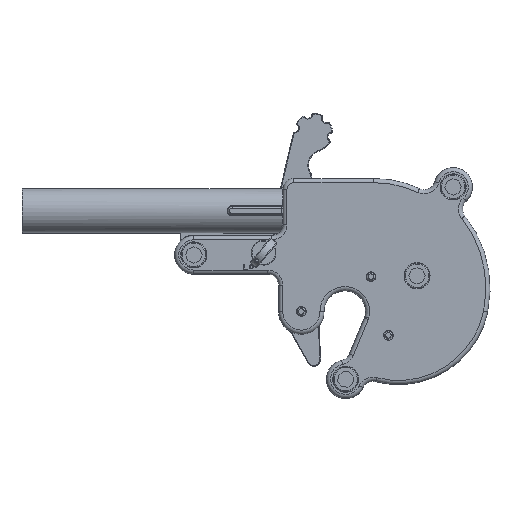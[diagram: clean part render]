
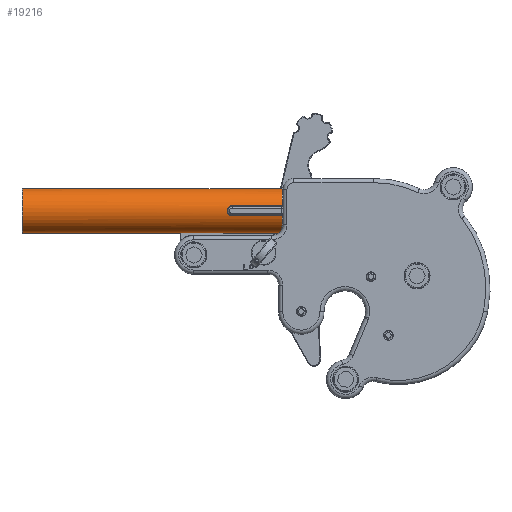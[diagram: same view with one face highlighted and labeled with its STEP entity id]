
A CAD part, top view. The second image highlights one B-rep face of the part: STEP entity #19216.
In plain terms, the highlighted cylindrical face has radius 8.1 mm (diameter 16.2 mm), a partial arc.
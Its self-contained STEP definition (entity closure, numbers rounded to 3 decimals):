
#982=CYLINDRICAL_SURFACE($,#20896,8.1);
#1768=B_SPLINE_CURVE_WITH_KNOTS($,3,(#31391,#31392,#31393,#31394,#31395,
#31396,#31397,#31398),.UNSPECIFIED.,.F.,.F.,(4,1,1,1,1,4),(5.289,
5.588,5.737,6.036,6.111,6.296),
 .UNSPECIFIED.);
#1769=B_SPLINE_CURVE_WITH_KNOTS($,3,(#31400,#31401,#31402,#31403),
 .UNSPECIFIED.,.F.,.F.,(4,4),(6.296,6.3),
 .UNSPECIFIED.);
#1772=B_SPLINE_CURVE_WITH_KNOTS($,3,(#31496,#31497,#31498,#31499,#31500,
#31501,#31502,#31503,#31504,#31505),.UNSPECIFIED.,.F.,.F.,(4,1,1,1,1,1,
1,4),(0.,0.079,0.118,0.236,0.315,
0.394,0.473,0.552),.UNSPECIFIED.);
#1778=B_SPLINE_CURVE_WITH_KNOTS($,3,(#31861,#31862,#31863,#31864,#31865,
#31866),.UNSPECIFIED.,.F.,.F.,(4,2,4),(-0.162,-0.152,
-0.143),.UNSPECIFIED.);
#1779=B_SPLINE_CURVE_WITH_KNOTS($,3,(#31923,#31924,#31925,#31926,#31927,
#31928,#31929,#31930,#31931,#31932),.UNSPECIFIED.,.F.,.F.,(4,2,2,2,4),(0.,
0.,0.04,0.052,0.06),
 .UNSPECIFIED.);
#2176=FACE_OUTER_BOUND($,#3521,.T.);
#3521=EDGE_LOOP($,(#14006,#14007,#14008,#14009,#14010,#14011,#14012,#14013,
#14014,#14015,#14016,#14017,#14018,#14019));
#4990=CIRCLE($,#20615,8.1);
#5063=CIRCLE($,#20723,8.1);
#5080=CIRCLE($,#20748,8.1);
#5157=CIRCLE($,#20886,8.1);
#6527=LINE($,#30896,#7532);
#6555=LINE($,#31431,#7560);
#6557=LINE($,#31507,#7562);
#6607=LINE($,#32069,#7612);
#6608=LINE($,#32071,#7613);
#7532=VECTOR($,#23895,94.5);
#7560=VECTOR($,#24139,18.25);
#7562=VECTOR($,#24145,18.25);
#7612=VECTOR($,#24515,57.073);
#7613=VECTOR($,#24518,36.084);
#8621=VERTEX_POINT($,#30821);
#8622=VERTEX_POINT($,#30825);
#8636=VERTEX_POINT($,#30895);
#8709=VERTEX_POINT($,#31329);
#8712=VERTEX_POINT($,#31336);
#8715=VERTEX_POINT($,#31390);
#8716=VERTEX_POINT($,#31399);
#8719=VERTEX_POINT($,#31421);
#8723=VERTEX_POINT($,#31429);
#8725=VERTEX_POINT($,#31494);
#8766=VERTEX_POINT($,#31855);
#8773=VERTEX_POINT($,#31921);
#8774=VERTEX_POINT($,#31922);
#8791=VERTEX_POINT($,#32056);
#10437=EDGE_CURVE($,#8622,#8621,#4990,.T.);
#10454=EDGE_CURVE($,#8621,#8636,#6527,.T.);
#10565=EDGE_CURVE($,#8709,#8712,#5063,.T.);
#10567=EDGE_CURVE($,#8712,#8715,#1768,.T.);
#10568=EDGE_CURVE($,#8715,#8716,#1769,.T.);
#10577=EDGE_CURVE($,#8723,#8709,#6555,.T.);
#10581=EDGE_CURVE($,#8725,#8723,#1772,.T.);
#10582=EDGE_CURVE($,#8719,#8725,#6557,.T.);
#10592=EDGE_CURVE($,#8636,#8719,#5080,.T.);
#10669=EDGE_CURVE($,#8716,#8766,#1778,.T.);
#10680=EDGE_CURVE($,#8773,#8774,#1779,.F.);
#10729=EDGE_CURVE($,#8774,#8791,#5157,.T.);
#10736=EDGE_CURVE($,#8622,#8791,#6607,.T.);
#10737=EDGE_CURVE($,#8773,#8766,#6608,.T.);
#14006=ORIENTED_EDGE($,*,*,#10437,.F.);
#14007=ORIENTED_EDGE($,*,*,#10736,.T.);
#14008=ORIENTED_EDGE($,*,*,#10729,.F.);
#14009=ORIENTED_EDGE($,*,*,#10680,.F.);
#14010=ORIENTED_EDGE($,*,*,#10737,.T.);
#14011=ORIENTED_EDGE($,*,*,#10669,.F.);
#14012=ORIENTED_EDGE($,*,*,#10568,.F.);
#14013=ORIENTED_EDGE($,*,*,#10567,.F.);
#14014=ORIENTED_EDGE($,*,*,#10565,.F.);
#14015=ORIENTED_EDGE($,*,*,#10577,.F.);
#14016=ORIENTED_EDGE($,*,*,#10581,.F.);
#14017=ORIENTED_EDGE($,*,*,#10582,.F.);
#14018=ORIENTED_EDGE($,*,*,#10592,.F.);
#14019=ORIENTED_EDGE($,*,*,#10454,.F.);
#19216=ADVANCED_FACE($,(#2176),#982,.T.);
#20615=AXIS2_PLACEMENT_3D($,#30827,#23868,#23869);
#20723=AXIS2_PLACEMENT_3D($,#31340,#24117,#24118);
#20748=AXIS2_PLACEMENT_3D($,#31525,#24171,#24172);
#20886=AXIS2_PLACEMENT_3D($,#32057,#24495,#24496);
#20896=AXIS2_PLACEMENT_3D($,#32070,#24516,#24517);
#23868=DIRECTION('center_axis',(0.,0.,-1.));
#23869=DIRECTION('ref_axis',(-0.998,-0.067,0.));
#23895=DIRECTION($,(0.,0.,1.));
#24117=DIRECTION('center_axis',(0.,0.,1.));
#24118=DIRECTION('ref_axis',(-0.908,-0.419,0.));
#24139=DIRECTION($,(0.,0.,1.));
#24145=DIRECTION($,(0.,0.,-1.));
#24171=DIRECTION('center_axis',(0.,0.,1.));
#24172=DIRECTION('ref_axis',(-0.302,0.953,0.));
#24495=DIRECTION('center_axis',(0.,0.,1.));
#24496=DIRECTION('ref_axis',(0.604,-0.797,0.));
#24515=DIRECTION($,(0.,0.,1.));
#24516=DIRECTION('center_axis',(0.,0.,1.));
#24517=DIRECTION('ref_axis',(0.696,0.718,0.));
#24518=DIRECTION($,(0.,0.,1.));
#30821=CARTESIAN_POINT('',(-0.654,7.295,5.25));
#30825=CARTESIAN_POINT('',(0.077,-3.521,5.25));
#30827=CARTESIAN_POINT('Origin',(-6.294,1.481,5.25));
#30895=CARTESIAN_POINT('',(-0.654,7.295,99.75));
#30896=CARTESIAN_POINT($,(-0.654,7.295,0.));
#31329=CARTESIAN_POINT('',(-14.19,-0.325,99.75));
#31336=CARTESIAN_POINT('',(-12.464,-3.767,99.75));
#31340=CARTESIAN_POINT('Origin',(-6.294,1.481,99.75));
#31390=CARTESIAN_POINT('',(-3.194,-6.002,99.061));
#31391=CARTESIAN_POINT('Ctrl Pts',(-12.464,-3.767,
99.75));
#31392=CARTESIAN_POINT('Ctrl Pts',(-11.798,-4.55,
99.75));
#31393=CARTESIAN_POINT('Ctrl Pts',(-10.589,-5.508,99.421));
#31394=CARTESIAN_POINT('Ctrl Pts',(-8.314,-6.473,
98.73));
#31395=CARTESIAN_POINT('Ctrl Pts',(-6.5,-6.703,
98.442));
#31396=CARTESIAN_POINT('Ctrl Pts',(-4.597,-6.477,
98.685));
#31397=CARTESIAN_POINT('Ctrl Pts',(-3.761,-6.237,
98.901));
#31398=CARTESIAN_POINT('Ctrl Pts',(-3.194,-6.002,
99.061));
#31399=CARTESIAN_POINT('',(-3.154,-5.985,99.073));
#31400=CARTESIAN_POINT('Ctrl Pts',(-3.194,-6.002,99.061));
#31401=CARTESIAN_POINT('Ctrl Pts',(-3.181,-5.997,
99.065));
#31402=CARTESIAN_POINT('Ctrl Pts',(-3.167,-5.991,
99.069));
#31403=CARTESIAN_POINT('Ctrl Pts',(-3.154,-5.985,
99.073));
#31421=CARTESIAN_POINT('',(-14.19,3.287,99.75));
#31429=CARTESIAN_POINT('',(-14.19,-0.325,81.5));
#31431=CARTESIAN_POINT($,(-14.19,-0.325,0.));
#31494=CARTESIAN_POINT('',(-14.19,3.287,81.5));
#31496=CARTESIAN_POINT('Ctrl Pts',(-14.19,3.287,81.5));
#31497=CARTESIAN_POINT('Ctrl Pts',(-14.19,3.287,81.237));
#31498=CARTESIAN_POINT('Ctrl Pts',(-14.213,3.193,80.845));
#31499=CARTESIAN_POINT('Ctrl Pts',(-14.299,2.761,80.176));
#31500=CARTESIAN_POINT('Ctrl Pts',(-14.398,2.039,79.735));
#31501=CARTESIAN_POINT('Ctrl Pts',(-14.397,1.063,79.736));
#31502=CARTESIAN_POINT('Ctrl Pts',(-14.319,0.316,
80.086));
#31503=CARTESIAN_POINT('Ctrl Pts',(-14.221,-0.2,
80.713));
#31504=CARTESIAN_POINT('Ctrl Pts',(-14.19,-0.325,81.237));
#31505=CARTESIAN_POINT('Ctrl Pts',(-14.19,-0.325,81.5));
#31507=CARTESIAN_POINT($,(-14.19,3.287,0.));
#31525=CARTESIAN_POINT('Origin',(-6.294,1.481,99.75));
#31855=CARTESIAN_POINT('',(-3.194,-6.002,98.884));
#31861=CARTESIAN_POINT('Ctrl Pts',(-3.154,-5.985,
99.073));
#31862=CARTESIAN_POINT('Ctrl Pts',(-3.167,-5.991,
99.042));
#31863=CARTESIAN_POINT('Ctrl Pts',(-3.178,-5.995,
99.009));
#31864=CARTESIAN_POINT('Ctrl Pts',(-3.191,-6.001,
98.945));
#31865=CARTESIAN_POINT('Ctrl Pts',(-3.194,-6.002,98.914));
#31866=CARTESIAN_POINT('Ctrl Pts',(-3.194,-6.002,98.884));
#31921=CARTESIAN_POINT('',(-3.194,-6.002,62.8));
#31922=CARTESIAN_POINT('',(-2.838,-5.844,62.323));
#31923=CARTESIAN_POINT('Ctrl Pts',(-2.838,-5.844,
62.323));
#31924=CARTESIAN_POINT('Ctrl Pts',(-2.838,-5.845,
62.324));
#31925=CARTESIAN_POINT('Ctrl Pts',(-2.839,-5.845,
62.325));
#31926=CARTESIAN_POINT('Ctrl Pts',(-2.925,-5.886,
62.418));
#31927=CARTESIAN_POINT('Ctrl Pts',(-3.032,-5.934,
62.484));
#31928=CARTESIAN_POINT('Ctrl Pts',(-3.134,-5.977,
62.613));
#31929=CARTESIAN_POINT('Ctrl Pts',(-3.16,-5.988,
62.653));
#31930=CARTESIAN_POINT('Ctrl Pts',(-3.188,-6.,
62.732));
#31931=CARTESIAN_POINT('Ctrl Pts',(-3.194,-6.002,62.766));
#31932=CARTESIAN_POINT('Ctrl Pts',(-3.194,-6.002,62.8));
#32056=CARTESIAN_POINT('',(0.077,-3.521,62.323));
#32057=CARTESIAN_POINT('Origin',(-6.294,1.481,62.323));
#32069=CARTESIAN_POINT($,(0.077,-3.521,0.));
#32070=CARTESIAN_POINT('Origin',(-6.294,1.481,0.));
#32071=CARTESIAN_POINT($,(-3.194,-6.002,0.));
